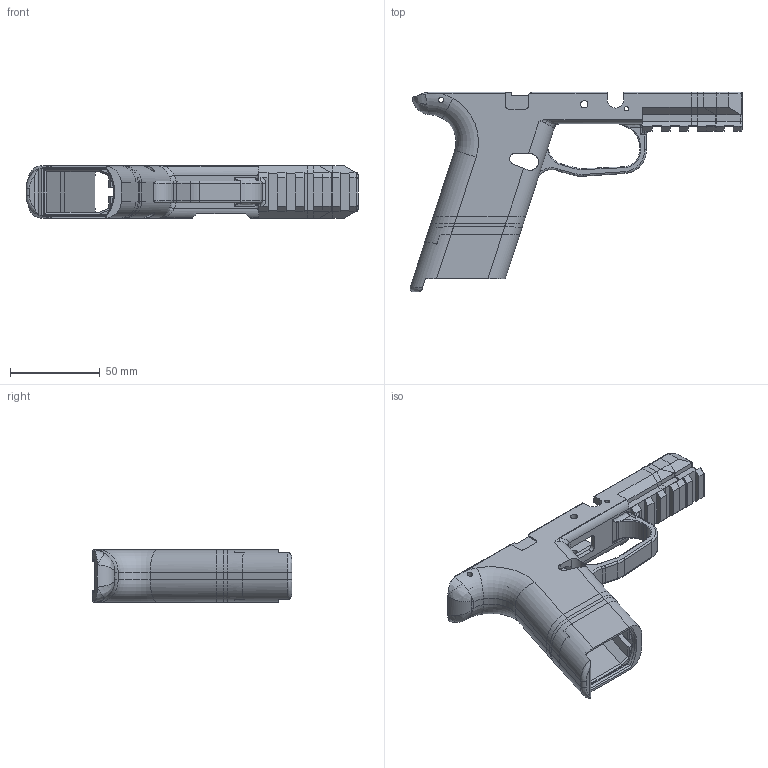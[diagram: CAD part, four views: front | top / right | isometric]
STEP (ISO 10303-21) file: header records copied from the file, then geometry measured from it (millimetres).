
FILE_DESCRIPTION(/* description */ (''),/* implementation_level */ '2;1');
FILE_NAME(/* name */ 'FNS-940.step',/* time_stamp */ '2021-05-28T01:25:09-04:00',/* author */ (''),/* organization */ (''),/* preprocessor_version */ 'ST-DEVELOPER v18.1',/* originating_system */ 'Autodesk Translation Framework v10.6.0.1341',/* authorisation */ '');
FILE_SCHEMA (('AUTOMOTIVE_DESIGN { 1 0 10303 214 3 1 1 }'));
Length unit declared in the file: millimetre
Products named in the file (5): FNS-9/40; Main Frame; Compact Size Grip; Standard Size Grip; Standard Size Grip (Stopgap)
Assembly tree (4 placements, depth 2):
  FNS-9/40
    Main Frame
    Compact Size Grip
    Standard Size Grip
    Standard Size Grip (Stopgap)
Bounding box: 184.47 x 110.97 x 29 mm (x, y, z)
Volume: 93505.4 mm3; surface area: 54404.5 mm2
Topology: 7 solids, 7 shells, 553 faces, 1537 edges, 986 vertices
Faces by surface type: plane 343, cylinder 149, bspline 28, torus 27, cone 6
Full cylindrical faces by diameter (mm): 2.5 x2, 3 x2, 4.1 x2
Entity records: 19178 total; most frequent: CARTESIAN_POINT 4863, ORIENTED_EDGE 3070, DIRECTION 2848, EDGE_CURVE 1535, LINE 1066, VECTOR 1066, VERTEX_POINT 986, AXIS2_PLACEMENT_3D 891
